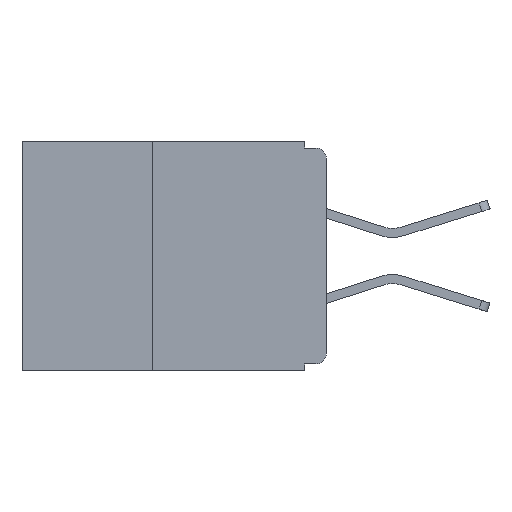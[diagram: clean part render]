
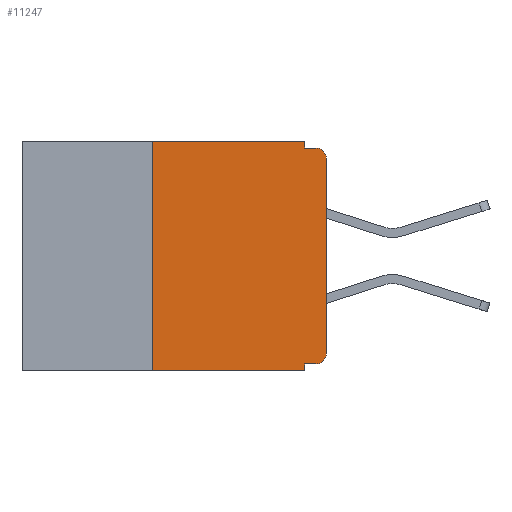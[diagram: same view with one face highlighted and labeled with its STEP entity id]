
A CAD part, left-side view. The second image highlights one B-rep face of the part: STEP entity #11247.
In plain terms, the highlighted planar face has unit normal (-1, 0, 0).
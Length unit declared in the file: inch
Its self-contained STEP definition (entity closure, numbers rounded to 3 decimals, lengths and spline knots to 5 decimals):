
#7 = LINE ( 'NONE', #6937, #13039 ) ;
#162 = VERTEX_POINT ( 'NONE', #18003 ) ;
#283 = ORIENTED_EDGE ( 'NONE', *, *, #16075, .F. ) ;
#346 = CARTESIAN_POINT ( 'NONE',  ( 0., 0.437, -0.33 ) ) ;
#492 = CARTESIAN_POINT ( 'NONE',  ( 0., 0.031, -0.32 ) ) ;
#1180 = VERTEX_POINT ( 'NONE', #1876 ) ;
#1361 = VECTOR ( 'NONE', #10101, 39.37008 ) ;
#1380 = DIRECTION ( 'NONE',  ( 0., 0., -1. ) ) ;
#1472 = EDGE_CURVE ( 'NONE', #1180, #7157, #4528, .T. ) ;
#1876 = CARTESIAN_POINT ( 'NONE',  ( 0., 0., -0.305 ) ) ;
#2022 = CIRCLE ( 'NONE', #15518, 0.015 ) ;
#2045 = DIRECTION ( 'NONE',  ( -1., 0., 0. ) ) ;
#2143 = VECTOR ( 'NONE', #17827, 39.37008 ) ;
#2855 = EDGE_LOOP ( 'NONE', ( #21703, #12374, #3848, #15643, #19435, #283, #10439, #11161, #8616, #13358 ) ) ;
#3008 = VERTEX_POINT ( 'NONE', #19224 ) ;
#3542 = VECTOR ( 'NONE', #7951, 39.37008 ) ;
#3614 = CARTESIAN_POINT ( 'NONE',  ( 0., 0.015, -0.32 ) ) ;
#3848 = ORIENTED_EDGE ( 'NONE', *, *, #16654, .F. ) ;
#4072 = EDGE_CURVE ( 'NONE', #4675, #15598, #7087, .T. ) ;
#4354 = LINE ( 'NONE', #7856, #12922 ) ;
#4528 = LINE ( 'NONE', #11720, #21524 ) ;
#4675 = VERTEX_POINT ( 'NONE', #3614 ) ;
#5834 = PLANE ( 'NONE',  #8493 ) ;
#6353 = DIRECTION ( 'NONE',  ( 0., -1., 0. ) ) ;
#6937 = CARTESIAN_POINT ( 'NONE',  ( 0., 0.437, 0. ) ) ;
#7087 = LINE ( 'NONE', #17508, #2143 ) ;
#7157 = VERTEX_POINT ( 'NONE', #9934 ) ;
#7655 = EDGE_CURVE ( 'NONE', #7851, #19872, #7, .T. ) ;
#7777 = AXIS2_PLACEMENT_3D ( 'NONE', #21596, #11521, #1380 ) ;
#7851 = VERTEX_POINT ( 'NONE', #20833 ) ;
#7856 = CARTESIAN_POINT ( 'NONE',  ( 0., 0., -0.01 ) ) ;
#7951 = DIRECTION ( 'NONE',  ( 0., 0., 1. ) ) ;
#8282 = LINE ( 'NONE', #19290, #16876 ) ;
#8493 = AXIS2_PLACEMENT_3D ( 'NONE', #17766, #19485, #9241 ) ;
#8616 = ORIENTED_EDGE ( 'NONE', *, *, #4072, .F. ) ;
#9241 = DIRECTION ( 'NONE',  ( 0., 0., -1. ) ) ;
#9934 = CARTESIAN_POINT ( 'NONE',  ( 0., 0., -0.025 ) ) ;
#10101 = DIRECTION ( 'NONE',  ( 0., 0., -1. ) ) ;
#10439 = ORIENTED_EDGE ( 'NONE', *, *, #14963, .T. ) ;
#10680 = VERTEX_POINT ( 'NONE', #14355 ) ;
#10898 = DIRECTION ( 'NONE',  ( 0., 0., 1. ) ) ;
#11161 = ORIENTED_EDGE ( 'NONE', *, *, #12647, .F. ) ;
#11247 = ADVANCED_FACE ( 'NONE', ( #19164 ), #5834, .F. ) ;
#11521 = DIRECTION ( 'NONE',  ( -1., 0., 0. ) ) ;
#11720 = CARTESIAN_POINT ( 'NONE',  ( 0., 0., 0. ) ) ;
#12200 = CARTESIAN_POINT ( 'NONE',  ( 0., 0.015, -0.305 ) ) ;
#12374 = ORIENTED_EDGE ( 'NONE', *, *, #20460, .T. ) ;
#12526 = CIRCLE ( 'NONE', #7777, 0.015 ) ;
#12647 = EDGE_CURVE ( 'NONE', #15598, #162, #14904, .T. ) ;
#12922 = VECTOR ( 'NONE', #18168, 39.37008 ) ;
#13039 = VECTOR ( 'NONE', #6353, 39.37008 ) ;
#13090 = CARTESIAN_POINT ( 'NONE',  ( 0., 0.25, -0.33 ) ) ;
#13358 = ORIENTED_EDGE ( 'NONE', *, *, #18187, .T. ) ;
#13931 = DIRECTION ( 'NONE',  ( 0., 0., -1. ) ) ;
#14355 = CARTESIAN_POINT ( 'NONE',  ( 0., 0.031, -0.01 ) ) ;
#14904 = LINE ( 'NONE', #18606, #1361 ) ;
#14963 = EDGE_CURVE ( 'NONE', #3008, #162, #20332, .T. ) ;
#15337 = VECTOR ( 'NONE', #17267, 39.37008 ) ;
#15518 = AXIS2_PLACEMENT_3D ( 'NONE', #12200, #2045, #13931 ) ;
#15598 = VERTEX_POINT ( 'NONE', #492 ) ;
#15643 = ORIENTED_EDGE ( 'NONE', *, *, #18313, .F. ) ;
#16075 = EDGE_CURVE ( 'NONE', #3008, #7851, #17628, .T. ) ;
#16654 = EDGE_CURVE ( 'NONE', #10680, #20993, #4354, .T. ) ;
#16876 = VECTOR ( 'NONE', #20974, 39.37008 ) ;
#17267 = DIRECTION ( 'NONE',  ( 0., -1., 0. ) ) ;
#17508 = CARTESIAN_POINT ( 'NONE',  ( 0., 0., -0.32 ) ) ;
#17628 = LINE ( 'NONE', #13090, #3542 ) ;
#17766 = CARTESIAN_POINT ( 'NONE',  ( 0., 0.437, 0. ) ) ;
#17827 = DIRECTION ( 'NONE',  ( 0., 1., 0. ) ) ;
#18003 = CARTESIAN_POINT ( 'NONE',  ( 0., 0.031, -0.33 ) ) ;
#18168 = DIRECTION ( 'NONE',  ( 0., -1., 0. ) ) ;
#18187 = EDGE_CURVE ( 'NONE', #4675, #1180, #2022, .T. ) ;
#18227 = CARTESIAN_POINT ( 'NONE',  ( 0., 0.015, -0.01 ) ) ;
#18313 = EDGE_CURVE ( 'NONE', #19872, #10680, #8282, .T. ) ;
#18606 = CARTESIAN_POINT ( 'NONE',  ( 0., 0.031, -0.33 ) ) ;
#19164 = FACE_OUTER_BOUND ( 'NONE', #2855, .T. ) ;
#19224 = CARTESIAN_POINT ( 'NONE',  ( 0., 0.25, -0.33 ) ) ;
#19290 = CARTESIAN_POINT ( 'NONE',  ( 0., 0.031, 0. ) ) ;
#19435 = ORIENTED_EDGE ( 'NONE', *, *, #7655, .F. ) ;
#19485 = DIRECTION ( 'NONE',  ( 1., 0., 0. ) ) ;
#19872 = VERTEX_POINT ( 'NONE', #21744 ) ;
#20332 = LINE ( 'NONE', #346, #15337 ) ;
#20460 = EDGE_CURVE ( 'NONE', #7157, #20993, #12526, .T. ) ;
#20833 = CARTESIAN_POINT ( 'NONE',  ( 0., 0.25, 0. ) ) ;
#20974 = DIRECTION ( 'NONE',  ( 0., 0., -1. ) ) ;
#20993 = VERTEX_POINT ( 'NONE', #18227 ) ;
#21524 = VECTOR ( 'NONE', #10898, 39.37008 ) ;
#21596 = CARTESIAN_POINT ( 'NONE',  ( 0., 0.015, -0.025 ) ) ;
#21703 = ORIENTED_EDGE ( 'NONE', *, *, #1472, .T. ) ;
#21744 = CARTESIAN_POINT ( 'NONE',  ( 0., 0.031, 0. ) ) ;
